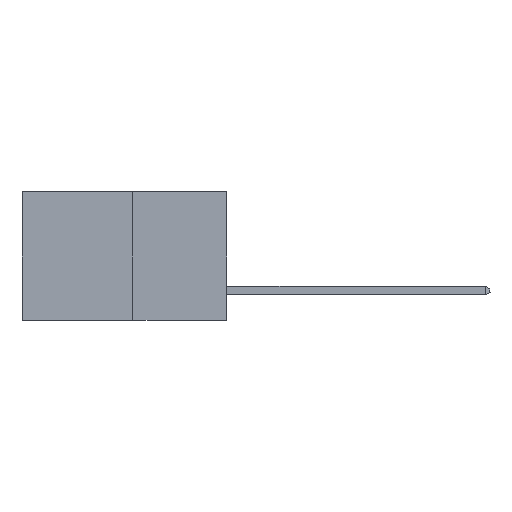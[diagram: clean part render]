
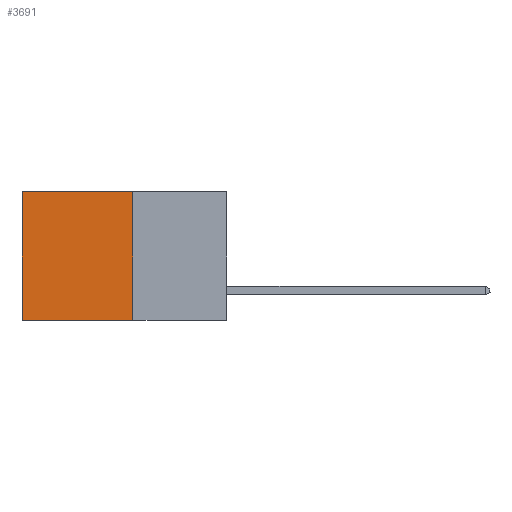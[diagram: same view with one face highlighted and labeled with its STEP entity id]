
A CAD part, left-side view. The second image highlights one B-rep face of the part: STEP entity #3691.
In plain terms, the highlighted planar face has unit normal (-1, 0, 0).
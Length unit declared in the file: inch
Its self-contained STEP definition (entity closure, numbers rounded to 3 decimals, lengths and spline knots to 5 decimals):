
#554 = DIRECTION ( 'NONE',  ( 0., 1., 0. ) ) ;
#1165 = AXIS2_PLACEMENT_3D ( 'NONE', #31701, #24281, #9349 ) ;
#1610 = FACE_OUTER_BOUND ( 'NONE', #2576, .T. ) ;
#2576 = EDGE_LOOP ( 'NONE', ( #23892, #7384, #28730, #23099 ) ) ;
#2726 = LINE ( 'NONE', #10358, #15210 ) ;
#3257 = LINE ( 'NONE', #11891, #9087 ) ;
#3691 = ADVANCED_FACE ( 'NONE', ( #1610 ), #29171, .F. ) ;
#5156 = VECTOR ( 'NONE', #8706, 39.37008 ) ;
#6146 = LINE ( 'NONE', #30443, #18647 ) ;
#6881 = VERTEX_POINT ( 'NONE', #24015 ) ;
#7384 = ORIENTED_EDGE ( 'NONE', *, *, #20406, .F. ) ;
#7872 = DIRECTION ( 'NONE',  ( 0., 0., -1. ) ) ;
#8706 = DIRECTION ( 'NONE',  ( 0., 1., 0. ) ) ;
#9087 = VECTOR ( 'NONE', #26805, 39.37008 ) ;
#9349 = DIRECTION ( 'NONE',  ( 0., 0., -1. ) ) ;
#10358 = CARTESIAN_POINT ( 'NONE',  ( 0.277, 0.27, -0.37 ) ) ;
#11767 = LINE ( 'NONE', #31044, #5156 ) ;
#11891 = CARTESIAN_POINT ( 'NONE',  ( 0.277, 0.59, -0.37 ) ) ;
#12292 = VERTEX_POINT ( 'NONE', #17851 ) ;
#14448 = CARTESIAN_POINT ( 'NONE',  ( 0.277, 0.59, -0.37 ) ) ;
#15210 = VECTOR ( 'NONE', #7872, 39.37008 ) ;
#16190 = VERTEX_POINT ( 'NONE', #19069 ) ;
#17851 = CARTESIAN_POINT ( 'NONE',  ( 0.277, 0.27, 0. ) ) ;
#18647 = VECTOR ( 'NONE', #554, 39.37008 ) ;
#19069 = CARTESIAN_POINT ( 'NONE',  ( 0.277, 0.27, -0.37 ) ) ;
#20108 = VERTEX_POINT ( 'NONE', #14448 ) ;
#20406 = EDGE_CURVE ( 'NONE', #16190, #20108, #6146, .T. ) ;
#23099 = ORIENTED_EDGE ( 'NONE', *, *, #27467, .T. ) ;
#23892 = ORIENTED_EDGE ( 'NONE', *, *, #32292, .T. ) ;
#24015 = CARTESIAN_POINT ( 'NONE',  ( 0.277, 0.59, 0. ) ) ;
#24281 = DIRECTION ( 'NONE',  ( 1., 0., 0. ) ) ;
#24718 = EDGE_CURVE ( 'NONE', #12292, #16190, #2726, .T. ) ;
#26805 = DIRECTION ( 'NONE',  ( 0., 0., -1. ) ) ;
#27467 = EDGE_CURVE ( 'NONE', #12292, #6881, #11767, .T. ) ;
#28730 = ORIENTED_EDGE ( 'NONE', *, *, #24718, .F. ) ;
#29171 = PLANE ( 'NONE',  #1165 ) ;
#30443 = CARTESIAN_POINT ( 'NONE',  ( 0.277, 0.27, -0.37 ) ) ;
#31044 = CARTESIAN_POINT ( 'NONE',  ( 0.277, 0.27, 0. ) ) ;
#31701 = CARTESIAN_POINT ( 'NONE',  ( 0.277, 0.27, -0.37 ) ) ;
#32292 = EDGE_CURVE ( 'NONE', #6881, #20108, #3257, .T. ) ;
